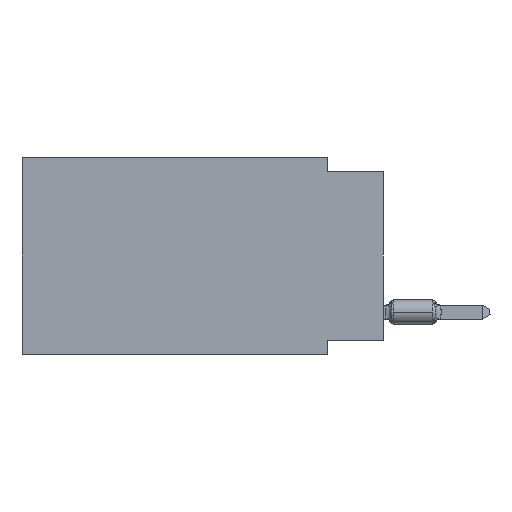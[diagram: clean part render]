
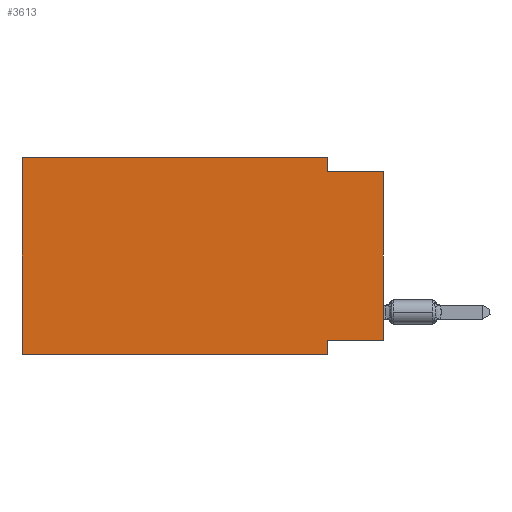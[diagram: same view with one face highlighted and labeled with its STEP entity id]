
A CAD part, left-side view. The second image highlights one B-rep face of the part: STEP entity #3613.
In plain terms, the highlighted planar face has unit normal (-1, 0, 0).
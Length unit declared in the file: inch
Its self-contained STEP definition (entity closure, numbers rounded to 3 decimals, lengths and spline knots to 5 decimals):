
#492 = CARTESIAN_POINT ( 'NONE',  ( 0., 0., -0.325 ) ) ;
#1169 = LINE ( 'NONE', #492, #29078 ) ;
#1412 = CARTESIAN_POINT ( 'NONE',  ( 0., 0.645, -0.35 ) ) ;
#3613 = ADVANCED_FACE ( 'NONE', ( #63173 ), #58023, .F. ) ;
#4804 = EDGE_CURVE ( 'NONE', #36611, #52189, #24069, .T. ) ;
#6486 = CARTESIAN_POINT ( 'NONE',  ( 0., 0.1, -0.325 ) ) ;
#9069 = CARTESIAN_POINT ( 'NONE',  ( 0., 0.1, 0. ) ) ;
#9276 = CARTESIAN_POINT ( 'NONE',  ( 0., 0.1, 0. ) ) ;
#9476 = DIRECTION ( 'NONE',  ( 0., 0., -1. ) ) ;
#10629 = DIRECTION ( 'NONE',  ( 0., -1., 0. ) ) ;
#10981 = CARTESIAN_POINT ( 'NONE',  ( 0., 0., -0.025 ) ) ;
#11172 = EDGE_CURVE ( 'NONE', #65105, #23354, #57446, .T. ) ;
#13260 = EDGE_CURVE ( 'NONE', #19482, #32515, #1169, .T. ) ;
#15072 = EDGE_CURVE ( 'NONE', #38471, #65105, #61043, .T. ) ;
#16329 = DIRECTION ( 'NONE',  ( 1., 0., 0. ) ) ;
#16411 = EDGE_LOOP ( 'NONE', ( #55395, #34193, #45863, #22312, #34368, #46208, #56373, #37992 ) ) ;
#17963 = EDGE_CURVE ( 'NONE', #52189, #38471, #58875, .T. ) ;
#18607 = CARTESIAN_POINT ( 'NONE',  ( 0., 0.645, 0. ) ) ;
#18862 = VECTOR ( 'NONE', #43178, 39.37008 ) ;
#18881 = VERTEX_POINT ( 'NONE', #34308 ) ;
#19254 = CARTESIAN_POINT ( 'NONE',  ( 0., 0., -0.325 ) ) ;
#19482 = VERTEX_POINT ( 'NONE', #19254 ) ;
#20689 = DIRECTION ( 'NONE',  ( 0., 1., 0. ) ) ;
#22312 = ORIENTED_EDGE ( 'NONE', *, *, #17963, .F. ) ;
#22992 = CARTESIAN_POINT ( 'NONE',  ( 0., 0., 0. ) ) ;
#23354 = VERTEX_POINT ( 'NONE', #52045 ) ;
#24069 = LINE ( 'NONE', #18607, #65777 ) ;
#24795 = DIRECTION ( 'NONE',  ( 0., 0., -1. ) ) ;
#27740 = DIRECTION ( 'NONE',  ( 0., -1., 0. ) ) ;
#29078 = VECTOR ( 'NONE', #20689, 39.37008 ) ;
#29603 = AXIS2_PLACEMENT_3D ( 'NONE', #40952, #16329, #61788 ) ;
#30367 = VECTOR ( 'NONE', #24795, 39.37008 ) ;
#32206 = DIRECTION ( 'NONE',  ( 0., -1., 0. ) ) ;
#32515 = VERTEX_POINT ( 'NONE', #6486 ) ;
#32748 = EDGE_CURVE ( 'NONE', #36611, #18881, #38035, .T. ) ;
#34193 = ORIENTED_EDGE ( 'NONE', *, *, #11172, .F. ) ;
#34308 = CARTESIAN_POINT ( 'NONE',  ( 0., 0.1, -0.35 ) ) ;
#34368 = ORIENTED_EDGE ( 'NONE', *, *, #4804, .F. ) ;
#36611 = VERTEX_POINT ( 'NONE', #43612 ) ;
#37992 = ORIENTED_EDGE ( 'NONE', *, *, #13260, .F. ) ;
#38035 = LINE ( 'NONE', #1412, #53734 ) ;
#38073 = LINE ( 'NONE', #22992, #18862 ) ;
#38471 = VERTEX_POINT ( 'NONE', #9276 ) ;
#40952 = CARTESIAN_POINT ( 'NONE',  ( 0., 0.645, 0. ) ) ;
#41392 = CARTESIAN_POINT ( 'NONE',  ( 0., 0.645, 0. ) ) ;
#41616 = CARTESIAN_POINT ( 'NONE',  ( 0., 0.1, -0.35 ) ) ;
#42161 = CARTESIAN_POINT ( 'NONE',  ( 0., 0.645, 0. ) ) ;
#43178 = DIRECTION ( 'NONE',  ( 0., 0., 1. ) ) ;
#43612 = CARTESIAN_POINT ( 'NONE',  ( 0., 0.645, -0.35 ) ) ;
#44541 = EDGE_CURVE ( 'NONE', #19482, #23354, #38073, .T. ) ;
#45863 = ORIENTED_EDGE ( 'NONE', *, *, #15072, .F. ) ;
#46208 = ORIENTED_EDGE ( 'NONE', *, *, #32748, .T. ) ;
#48646 = CARTESIAN_POINT ( 'NONE',  ( 0., 0.1, -0.025 ) ) ;
#49445 = EDGE_CURVE ( 'NONE', #32515, #18881, #57318, .T. ) ;
#49753 = VECTOR ( 'NONE', #27740, 39.37008 ) ;
#50715 = DIRECTION ( 'NONE',  ( 0., 0., 1. ) ) ;
#52045 = CARTESIAN_POINT ( 'NONE',  ( 0., 0., -0.025 ) ) ;
#52189 = VERTEX_POINT ( 'NONE', #41392 ) ;
#53734 = VECTOR ( 'NONE', #32206, 39.37008 ) ;
#55395 = ORIENTED_EDGE ( 'NONE', *, *, #44541, .T. ) ;
#56373 = ORIENTED_EDGE ( 'NONE', *, *, #49445, .F. ) ;
#57318 = LINE ( 'NONE', #41616, #59485 ) ;
#57446 = LINE ( 'NONE', #10981, #58386 ) ;
#58023 = PLANE ( 'NONE',  #29603 ) ;
#58386 = VECTOR ( 'NONE', #10629, 39.37008 ) ;
#58875 = LINE ( 'NONE', #42161, #49753 ) ;
#59485 = VECTOR ( 'NONE', #9476, 39.37008 ) ;
#61043 = LINE ( 'NONE', #9069, #30367 ) ;
#61788 = DIRECTION ( 'NONE',  ( 0., 0., -1. ) ) ;
#63173 = FACE_OUTER_BOUND ( 'NONE', #16411, .T. ) ;
#65105 = VERTEX_POINT ( 'NONE', #48646 ) ;
#65777 = VECTOR ( 'NONE', #50715, 39.37008 ) ;
